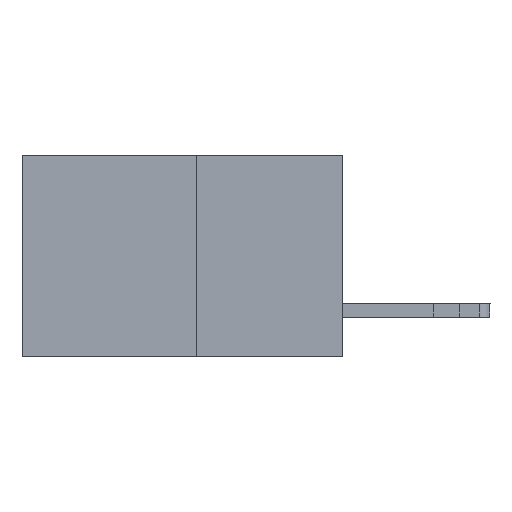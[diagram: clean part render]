
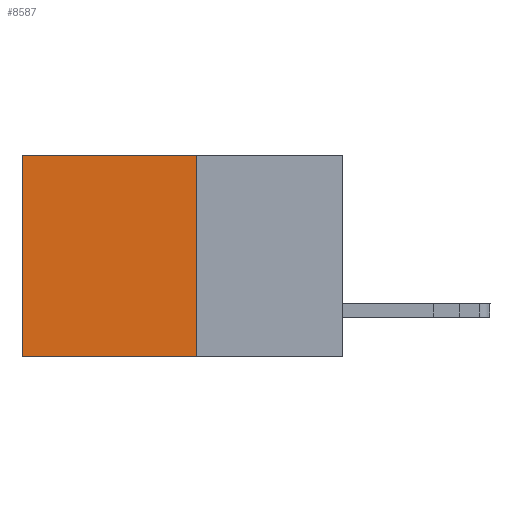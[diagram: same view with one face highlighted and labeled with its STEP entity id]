
A CAD part, left-side view. The second image highlights one B-rep face of the part: STEP entity #8587.
In plain terms, the highlighted planar face has unit normal (-1, 0, 0).
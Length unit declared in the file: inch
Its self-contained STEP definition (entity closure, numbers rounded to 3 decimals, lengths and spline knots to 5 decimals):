
#428 = DIRECTION ( 'NONE',  ( 0., 1., 0. ) ) ;
#1401 = CARTESIAN_POINT ( 'NONE',  ( 0.277, 0.27, -0.37 ) ) ;
#1515 = LINE ( 'NONE', #6807, #5021 ) ;
#1864 = ORIENTED_EDGE ( 'NONE', *, *, #8146, .F. ) ;
#2500 = CARTESIAN_POINT ( 'NONE',  ( 0.277, 0.59, -0.37 ) ) ;
#2583 = DIRECTION ( 'NONE',  ( 0., 0., -1. ) ) ;
#4480 = PLANE ( 'NONE',  #12182 ) ;
#4550 = DIRECTION ( 'NONE',  ( 1., 0., 0. ) ) ;
#4568 = DIRECTION ( 'NONE',  ( 0., 0., -1. ) ) ;
#5021 = VECTOR ( 'NONE', #15800, 39.37008 ) ;
#5045 = DIRECTION ( 'NONE',  ( 0., 0., -1. ) ) ;
#5598 = VECTOR ( 'NONE', #2583, 39.37008 ) ;
#6030 = FACE_OUTER_BOUND ( 'NONE', #9016, .T. ) ;
#6117 = CARTESIAN_POINT ( 'NONE',  ( 0.277, 0.27, -0.37 ) ) ;
#6133 = VERTEX_POINT ( 'NONE', #8118 ) ;
#6807 = CARTESIAN_POINT ( 'NONE',  ( 0.277, 0.27, 0. ) ) ;
#6976 = CARTESIAN_POINT ( 'NONE',  ( 0.277, 0.27, -0.37 ) ) ;
#7189 = VECTOR ( 'NONE', #428, 39.37008 ) ;
#7580 = EDGE_CURVE ( 'NONE', #12281, #6133, #1515, .T. ) ;
#7598 = LINE ( 'NONE', #6976, #7189 ) ;
#7606 = ORIENTED_EDGE ( 'NONE', *, *, #9754, .F. ) ;
#8118 = CARTESIAN_POINT ( 'NONE',  ( 0.277, 0.59, 0. ) ) ;
#8146 = EDGE_CURVE ( 'NONE', #12281, #10624, #16224, .T. ) ;
#8279 = VERTEX_POINT ( 'NONE', #2500 ) ;
#8587 = ADVANCED_FACE ( 'NONE', ( #6030 ), #4480, .F. ) ;
#8624 = LINE ( 'NONE', #10333, #5598 ) ;
#8780 = ORIENTED_EDGE ( 'NONE', *, *, #12687, .T. ) ;
#9016 = EDGE_LOOP ( 'NONE', ( #8780, #7606, #1864, #13171 ) ) ;
#9380 = CARTESIAN_POINT ( 'NONE',  ( 0.277, 0.27, 0. ) ) ;
#9754 = EDGE_CURVE ( 'NONE', #10624, #8279, #7598, .T. ) ;
#10333 = CARTESIAN_POINT ( 'NONE',  ( 0.277, 0.59, -0.37 ) ) ;
#10624 = VERTEX_POINT ( 'NONE', #6117 ) ;
#12182 = AXIS2_PLACEMENT_3D ( 'NONE', #1401, #4550, #4568 ) ;
#12281 = VERTEX_POINT ( 'NONE', #9380 ) ;
#12687 = EDGE_CURVE ( 'NONE', #6133, #8279, #8624, .T. ) ;
#13002 = VECTOR ( 'NONE', #5045, 39.37008 ) ;
#13171 = ORIENTED_EDGE ( 'NONE', *, *, #7580, .T. ) ;
#14915 = CARTESIAN_POINT ( 'NONE',  ( 0.277, 0.27, -0.37 ) ) ;
#15800 = DIRECTION ( 'NONE',  ( 0., 1., 0. ) ) ;
#16224 = LINE ( 'NONE', #14915, #13002 ) ;
